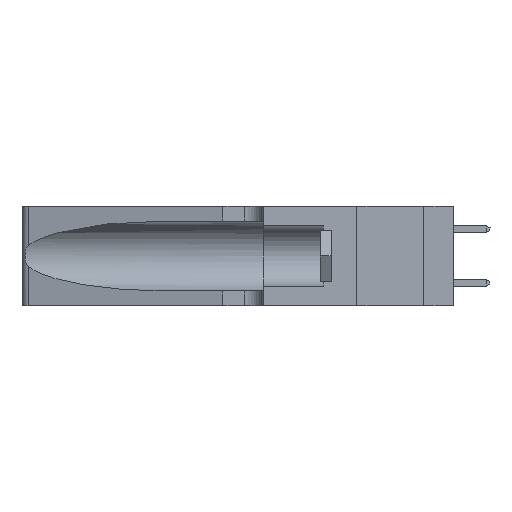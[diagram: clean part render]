
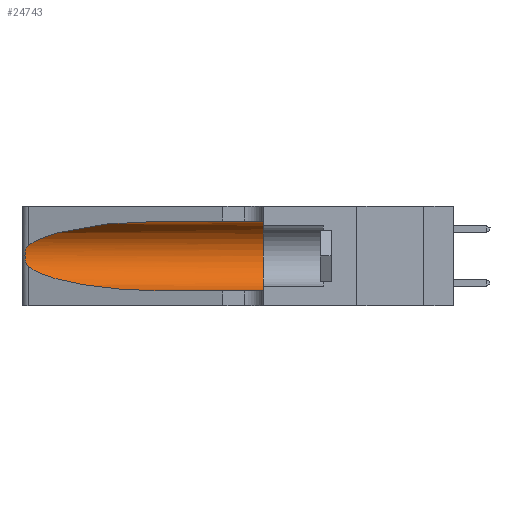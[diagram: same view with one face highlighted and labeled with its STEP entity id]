
A CAD part, left-side view. The second image highlights one B-rep face of the part: STEP entity #24743.
In plain terms, the highlighted cylindrical face has radius 3.308 mm (diameter 6.617 mm), a partial arc.
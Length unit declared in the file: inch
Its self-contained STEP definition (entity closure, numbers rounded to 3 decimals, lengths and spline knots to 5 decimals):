
#584 = EDGE_CURVE ( 'NONE', #41161, #35759, #32206, .T. ) ;
#674 = AXIS2_PLACEMENT_3D ( 'NONE', #15635, #38311, #18933 ) ;
#1055 = CARTESIAN_POINT ( 'NONE',  ( 0.25639, 1.23184, 0.21858 ) ) ;
#1594 = DIRECTION ( 'NONE',  ( 0., 0., -1. ) ) ;
#2565 = CARTESIAN_POINT ( 'NONE',  ( 0.25487, 1.22718, 0.22369 ) ) ;
#3199 = CARTESIAN_POINT ( 'NONE',  ( 0.1305, 0.72297, 0.05475 ) ) ;
#4123 = VECTOR ( 'NONE', #22389, 39.37008 ) ;
#4440 = CARTESIAN_POINT ( 'NONE',  ( 0.25854, 1.2359, 0.20912 ) ) ;
#4878 =( BOUNDED_CURVE ( )  B_SPLINE_CURVE ( 3, ( #42331, #39067, #22958, #3199 ),
 .UNSPECIFIED., .F., .F. ) 
 B_SPLINE_CURVE_WITH_KNOTS ( ( 4, 4 ),
 ( 3.44316, 4.71239 ),
 .UNSPECIFIED. ) 
 CURVE ( )  GEOMETRIC_REPRESENTATION_ITEM ( )  RATIONAL_B_SPLINE_CURVE ( ( 1., 0.87, 0.87, 1. ) ) 
 REPRESENTATION_ITEM ( '' )  );
#6417 = CYLINDRICAL_SURFACE ( 'NONE', #32437, 0.13025 ) ;
#7778 = CARTESIAN_POINT ( 'NONE',  ( 0.26075, 1.23896, 0.19203 ) ) ;
#7839 = ORIENTED_EDGE ( 'NONE', *, *, #40063, .F. ) ;
#8295 = CARTESIAN_POINT ( 'NONE',  ( 0.1305, 1.61858, 0.185 ) ) ;
#8648 = EDGE_CURVE ( 'NONE', #21456, #35759, #21684, .T. ) ;
#9835 = CARTESIAN_POINT ( 'NONE',  ( 0.1305, 0.35, 0.31525 ) ) ;
#11002 = VECTOR ( 'NONE', #11894, 39.37008 ) ;
#11129 = CARTESIAN_POINT ( 'NONE',  ( 0.26017, 1.23833, 0.17102 ) ) ;
#11571 = CARTESIAN_POINT ( 'NONE',  ( 0.25487, 1.22718, 0.14631 ) ) ;
#11894 = DIRECTION ( 'NONE',  ( 0., -1., 0. ) ) ;
#12476 = CARTESIAN_POINT ( 'NONE',  ( 0.1305, 0.72297, 0.31525 ) ) ;
#12798 = EDGE_LOOP ( 'NONE', ( #35853, #38934, #24785, #19201, #13589, #7839 ) ) ;
#13287 = EDGE_CURVE ( 'NONE', #24053, #21456, #4878, .T. ) ;
#13589 = ORIENTED_EDGE ( 'NONE', *, *, #584, .F. ) ;
#13873 = VERTEX_POINT ( 'NONE', #25585 ) ;
#14334 = CARTESIAN_POINT ( 'NONE',  ( 0.25555, 1.22994, 0.2215 ) ) ;
#14474 = CARTESIAN_POINT ( 'NONE',  ( 0.25789, 1.23486, 0.15765 ) ) ;
#15635 = CARTESIAN_POINT ( 'NONE',  ( 0.1305, 0.35, 0.185 ) ) ;
#16587 = CARTESIAN_POINT ( 'NONE',  ( 0.1305, 0.35, 0.05475 ) ) ;
#17754 = CARTESIAN_POINT ( 'NONE',  ( 0.25555, 1.22993, 0.14849 ) ) ;
#18933 = DIRECTION ( 'NONE',  ( 0., 0., 1. ) ) ;
#19118 = CARTESIAN_POINT ( 'NONE',  ( 0.1305, 1.61858, 0.05475 ) ) ;
#19201 = ORIENTED_EDGE ( 'NONE', *, *, #8648, .T. ) ;
#20965 = CARTESIAN_POINT ( 'NONE',  ( 0.1305, 0.72297, 0.31525 ) ) ;
#21456 = VERTEX_POINT ( 'NONE', #29030 ) ;
#21684 = LINE ( 'NONE', #19118, #4123 ) ;
#22358 = CARTESIAN_POINT ( 'NONE',  ( 0.2373, 1.15595, 0.28018 ) ) ;
#22389 = DIRECTION ( 'NONE',  ( 0., -1., 0. ) ) ;
#22958 = CARTESIAN_POINT ( 'NONE',  ( 0.18966, 0.96281, 0.05475 ) ) ;
#24053 = VERTEX_POINT ( 'NONE', #11571 ) ;
#24165 = CARTESIAN_POINT ( 'NONE',  ( 0.25787, 1.23484, 0.2124 ) ) ;
#24743 = ADVANCED_FACE ( 'NONE', ( #32521 ), #6417, .F. ) ;
#24785 = ORIENTED_EDGE ( 'NONE', *, *, #13287, .T. ) ;
#25585 = CARTESIAN_POINT ( 'NONE',  ( 0.25487, 1.22718, 0.22369 ) ) ;
#27400 = CARTESIAN_POINT ( 'NONE',  ( 0.26018, 1.23835, 0.19895 ) ) ;
#27894 = DIRECTION ( 'NONE',  ( 0., -1., 0. ) ) ;
#28123 = CARTESIAN_POINT ( 'NONE',  ( 0.1305, 1.61858, 0.31525 ) ) ;
#29030 = CARTESIAN_POINT ( 'NONE',  ( 0.1305, 0.72297, 0.05475 ) ) ;
#29043 = B_SPLINE_CURVE_WITH_KNOTS ( 'NONE', 3,
 ( #33759, #14334, #1055, #24165, #4440, #27400, #7778, #30662, #11129, #33899, #14474, #37141, #17754, #40427 ),
 .UNSPECIFIED., .F., .F.,
 ( 4, 2, 2, 2, 2, 2, 4 ),
 ( 0., 0.00027, 0.00053, 0.00107, 0.0016, 0.00187, 0.00214 ),
 .UNSPECIFIED. ) ;
#30662 = CARTESIAN_POINT ( 'NONE',  ( 0.26075, 1.23896, 0.178 ) ) ;
#32206 = CIRCLE ( 'NONE', #674, 0.13025 ) ;
#32437 = AXIS2_PLACEMENT_3D ( 'NONE', #8295, #27894, #1594 ) ;
#32521 = FACE_OUTER_BOUND ( 'NONE', #12798, .T. ) ;
#32910 = VERTEX_POINT ( 'NONE', #20965 ) ;
#33759 = CARTESIAN_POINT ( 'NONE',  ( 0.25487, 1.22718, 0.22369 ) ) ;
#33899 = CARTESIAN_POINT ( 'NONE',  ( 0.25856, 1.23593, 0.16098 ) ) ;
#35759 = VERTEX_POINT ( 'NONE', #16587 ) ;
#35853 = ORIENTED_EDGE ( 'NONE', *, *, #41008, .T. ) ;
#36550 =( BOUNDED_CURVE ( )  B_SPLINE_CURVE ( 3, ( #12476, #38456, #22358, #2565 ),
 .UNSPECIFIED., .F., .F. ) 
 B_SPLINE_CURVE_WITH_KNOTS ( ( 4, 4 ),
 ( 1.5708, 2.84003 ),
 .UNSPECIFIED. ) 
 CURVE ( )  GEOMETRIC_REPRESENTATION_ITEM ( )  RATIONAL_B_SPLINE_CURVE ( ( 1., 0.87, 0.87, 1. ) ) 
 REPRESENTATION_ITEM ( '' )  );
#37141 = CARTESIAN_POINT ( 'NONE',  ( 0.25639, 1.23186, 0.15144 ) ) ;
#37966 = LINE ( 'NONE', #28123, #11002 ) ;
#38311 = DIRECTION ( 'NONE',  ( 0., 1., 0. ) ) ;
#38456 = CARTESIAN_POINT ( 'NONE',  ( 0.18966, 0.96281, 0.31525 ) ) ;
#38934 = ORIENTED_EDGE ( 'NONE', *, *, #41416, .T. ) ;
#39067 = CARTESIAN_POINT ( 'NONE',  ( 0.2373, 1.15595, 0.08982 ) ) ;
#40063 = EDGE_CURVE ( 'NONE', #32910, #41161, #37966, .T. ) ;
#40427 = CARTESIAN_POINT ( 'NONE',  ( 0.25487, 1.22718, 0.14631 ) ) ;
#41008 = EDGE_CURVE ( 'NONE', #32910, #13873, #36550, .T. ) ;
#41161 = VERTEX_POINT ( 'NONE', #9835 ) ;
#41416 = EDGE_CURVE ( 'NONE', #13873, #24053, #29043, .T. ) ;
#42331 = CARTESIAN_POINT ( 'NONE',  ( 0.25487, 1.22718, 0.14631 ) ) ;
